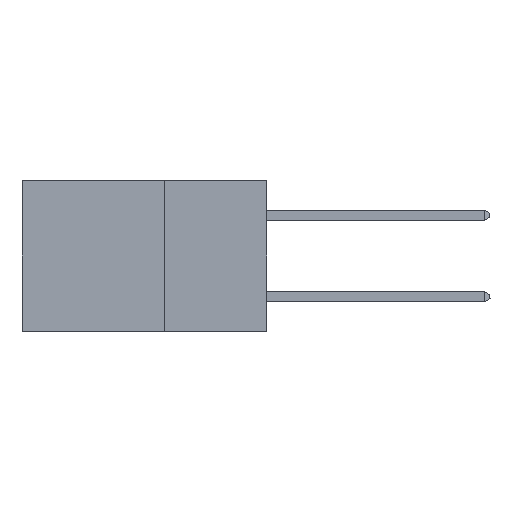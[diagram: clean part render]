
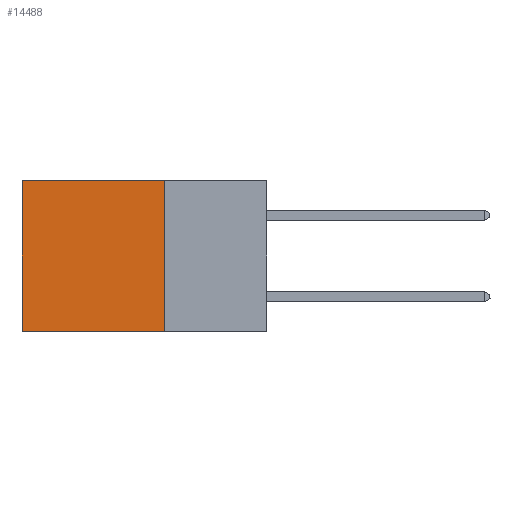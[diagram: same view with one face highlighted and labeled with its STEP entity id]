
A CAD part, left-side view. The second image highlights one B-rep face of the part: STEP entity #14488.
In plain terms, the highlighted planar face has unit normal (-1, 0, 0).
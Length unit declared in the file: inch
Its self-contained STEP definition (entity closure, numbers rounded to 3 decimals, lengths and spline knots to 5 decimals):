
#1672 = ORIENTED_EDGE ( 'NONE', *, *, #13360, .F. ) ;
#2974 = PLANE ( 'NONE',  #28316 ) ;
#4630 = CARTESIAN_POINT ( 'NONE',  ( 0.2875, 0.25, -0.37 ) ) ;
#5391 = CARTESIAN_POINT ( 'NONE',  ( 0.2875, 0.25, 0. ) ) ;
#5562 = VERTEX_POINT ( 'NONE', #5391 ) ;
#6237 = EDGE_CURVE ( 'NONE', #14298, #28352, #23930, .T. ) ;
#9091 = CARTESIAN_POINT ( 'NONE',  ( 0.2875, 0.25, 0. ) ) ;
#9345 = DIRECTION ( 'NONE',  ( 0., 1., 0. ) ) ;
#11617 = ORIENTED_EDGE ( 'NONE', *, *, #6237, .T. ) ;
#11682 = EDGE_CURVE ( 'NONE', #5562, #14298, #29276, .T. ) ;
#11720 = DIRECTION ( 'NONE',  ( 0., 0., -1. ) ) ;
#11969 = LINE ( 'NONE', #22709, #16345 ) ;
#12011 = VECTOR ( 'NONE', #18383, 39.37008 ) ;
#13360 = EDGE_CURVE ( 'NONE', #5562, #26165, #16827, .T. ) ;
#14298 = VERTEX_POINT ( 'NONE', #30746 ) ;
#14488 = ADVANCED_FACE ( 'NONE', ( #24412 ), #2974, .F. ) ;
#16345 = VECTOR ( 'NONE', #9345, 39.37008 ) ;
#16827 = LINE ( 'NONE', #9091, #29386 ) ;
#18383 = DIRECTION ( 'NONE',  ( 0., 1., 0. ) ) ;
#19927 = VECTOR ( 'NONE', #20759, 39.37008 ) ;
#20759 = DIRECTION ( 'NONE',  ( 0., 0., -1. ) ) ;
#21246 = CARTESIAN_POINT ( 'NONE',  ( 0.2875, 0.25, 0. ) ) ;
#21777 = ORIENTED_EDGE ( 'NONE', *, *, #34391, .F. ) ;
#22709 = CARTESIAN_POINT ( 'NONE',  ( 0.2875, 0.25, -0.37 ) ) ;
#23930 = LINE ( 'NONE', #34462, #19927 ) ;
#24412 = FACE_OUTER_BOUND ( 'NONE', #33632, .T. ) ;
#25650 = CARTESIAN_POINT ( 'NONE',  ( 0.2875, 0.25, 0. ) ) ;
#26165 = VERTEX_POINT ( 'NONE', #4630 ) ;
#26530 = DIRECTION ( 'NONE',  ( 1., 0., 0. ) ) ;
#27211 = DIRECTION ( 'NONE',  ( 0., 0., -1. ) ) ;
#27250 = CARTESIAN_POINT ( 'NONE',  ( 0.2875, 0.6, -0.37 ) ) ;
#28316 = AXIS2_PLACEMENT_3D ( 'NONE', #21246, #26530, #27211 ) ;
#28352 = VERTEX_POINT ( 'NONE', #27250 ) ;
#29276 = LINE ( 'NONE', #25650, #12011 ) ;
#29386 = VECTOR ( 'NONE', #11720, 39.37008 ) ;
#30746 = CARTESIAN_POINT ( 'NONE',  ( 0.2875, 0.6, 0. ) ) ;
#32563 = ORIENTED_EDGE ( 'NONE', *, *, #11682, .T. ) ;
#33632 = EDGE_LOOP ( 'NONE', ( #11617, #21777, #1672, #32563 ) ) ;
#34391 = EDGE_CURVE ( 'NONE', #26165, #28352, #11969, .T. ) ;
#34462 = CARTESIAN_POINT ( 'NONE',  ( 0.2875, 0.6, 0. ) ) ;
